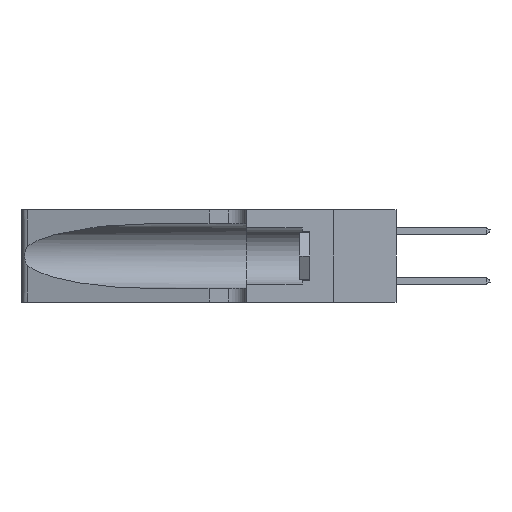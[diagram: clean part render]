
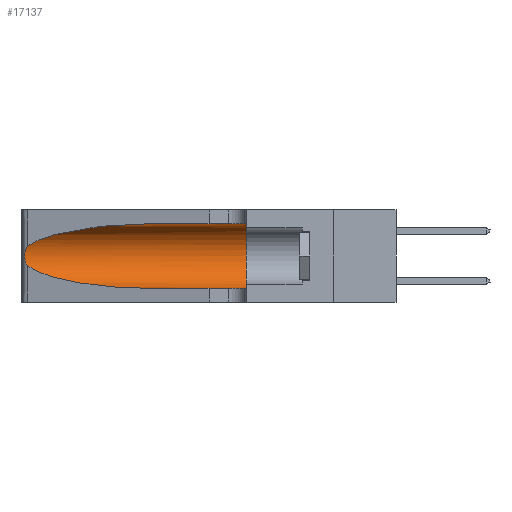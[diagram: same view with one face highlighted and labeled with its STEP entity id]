
A CAD part, left-side view. The second image highlights one B-rep face of the part: STEP entity #17137.
In plain terms, the highlighted cylindrical face has radius 3.308 mm (diameter 6.617 mm), a partial arc.
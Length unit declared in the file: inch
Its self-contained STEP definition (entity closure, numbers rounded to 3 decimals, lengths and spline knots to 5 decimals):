
#796 = ORIENTED_EDGE ( 'NONE', *, *, #6608, .F. ) ;
#1020 = CARTESIAN_POINT ( 'NONE',  ( 0.26018, 1.23835, 0.19895 ) ) ;
#1089 = CARTESIAN_POINT ( 'NONE',  ( 0.25789, 1.23486, 0.15765 ) ) ;
#1200 = ORIENTED_EDGE ( 'NONE', *, *, #15954, .F. ) ;
#2263 = EDGE_CURVE ( 'NONE', #7986, #12534, #7721, .T. ) ;
#2265 = ORIENTED_EDGE ( 'NONE', *, *, #20033, .T. ) ;
#2362 = CARTESIAN_POINT ( 'NONE',  ( 0.25487, 1.22718, 0.14631 ) ) ;
#2555 = ORIENTED_EDGE ( 'NONE', *, *, #2263, .T. ) ;
#2839 = CARTESIAN_POINT ( 'NONE',  ( 0.25487, 1.22718, 0.22369 ) ) ;
#4433 = CARTESIAN_POINT ( 'NONE',  ( 0.25639, 1.23186, 0.15144 ) ) ;
#4493 = CARTESIAN_POINT ( 'NONE',  ( 0.1305, 0.72297, 0.31525 ) ) ;
#4564 = CARTESIAN_POINT ( 'NONE',  ( 0.1305, 0.72297, 0.31525 ) ) ;
#5736 = VERTEX_POINT ( 'NONE', #21040 ) ;
#6012 = CARTESIAN_POINT ( 'NONE',  ( 0.25487, 1.22718, 0.14631 ) ) ;
#6132 = LINE ( 'NONE', #9287, #9793 ) ;
#6608 = EDGE_CURVE ( 'NONE', #20489, #16386, #6132, .T. ) ;
#6741 = CARTESIAN_POINT ( 'NONE',  ( 0.1305, 0.35, 0.185 ) ) ;
#7234 = CARTESIAN_POINT ( 'NONE',  ( 0.1305, 0.72297, 0.05475 ) ) ;
#7451 = AXIS2_PLACEMENT_3D ( 'NONE', #6741, #14644, #20525 ) ;
#7662 = ORIENTED_EDGE ( 'NONE', *, *, #10128, .T. ) ;
#7721 = LINE ( 'NONE', #16367, #12068 ) ;
#7777 = CARTESIAN_POINT ( 'NONE',  ( 0.25787, 1.23484, 0.2124 ) ) ;
#7986 = VERTEX_POINT ( 'NONE', #7234 ) ;
#9232 = CARTESIAN_POINT ( 'NONE',  ( 0.25555, 1.22994, 0.2215 ) ) ;
#9287 = CARTESIAN_POINT ( 'NONE',  ( 0.1305, 1.61858, 0.31525 ) ) ;
#9518 = CARTESIAN_POINT ( 'NONE',  ( 0.25639, 1.23184, 0.21858 ) ) ;
#9793 = VECTOR ( 'NONE', #10057, 39.37008 ) ;
#10057 = DIRECTION ( 'NONE',  ( 0., -1., 0. ) ) ;
#10128 = EDGE_CURVE ( 'NONE', #5736, #7986, #15803, .T. ) ;
#10881 = CARTESIAN_POINT ( 'NONE',  ( 0.26075, 1.23896, 0.178 ) ) ;
#11299 = CARTESIAN_POINT ( 'NONE',  ( 0.1305, 0.35, 0.31525 ) ) ;
#11866 = CARTESIAN_POINT ( 'NONE',  ( 0.1305, 1.61858, 0.185 ) ) ;
#12068 = VECTOR ( 'NONE', #21257, 39.37008 ) ;
#12501 = CARTESIAN_POINT ( 'NONE',  ( 0.25487, 1.22718, 0.22369 ) ) ;
#12534 = VERTEX_POINT ( 'NONE', #20187 ) ;
#12577 =( BOUNDED_CURVE ( )  B_SPLINE_CURVE ( 3, ( #4493, #19387, #19295, #2839 ),
 .UNSPECIFIED., .F., .F. ) 
 B_SPLINE_CURVE_WITH_KNOTS ( ( 4, 4 ),
 ( 1.5708, 2.84003 ),
 .UNSPECIFIED. ) 
 CURVE ( )  GEOMETRIC_REPRESENTATION_ITEM ( )  RATIONAL_B_SPLINE_CURVE ( ( 1., 0.87, 0.87, 1. ) ) 
 REPRESENTATION_ITEM ( '' )  );
#12721 = CARTESIAN_POINT ( 'NONE',  ( 0.25856, 1.23593, 0.16098 ) ) ;
#13360 = FACE_OUTER_BOUND ( 'NONE', #17793, .T. ) ;
#13927 = CARTESIAN_POINT ( 'NONE',  ( 0.1305, 0.72297, 0.05475 ) ) ;
#14201 = CARTESIAN_POINT ( 'NONE',  ( 0.26075, 1.23896, 0.19203 ) ) ;
#14422 = CARTESIAN_POINT ( 'NONE',  ( 0.25854, 1.2359, 0.20912 ) ) ;
#14644 = DIRECTION ( 'NONE',  ( 0., 1., 0. ) ) ;
#14737 = EDGE_CURVE ( 'NONE', #20489, #20979, #12577, .T. ) ;
#14991 = ORIENTED_EDGE ( 'NONE', *, *, #14737, .T. ) ;
#15296 = DIRECTION ( 'NONE',  ( 0., 0., -1. ) ) ;
#15533 = CARTESIAN_POINT ( 'NONE',  ( 0.25487, 1.22718, 0.22369 ) ) ;
#15803 =( BOUNDED_CURVE ( )  B_SPLINE_CURVE ( 3, ( #2362, #18840, #20323, #13927 ),
 .UNSPECIFIED., .F., .T. ) 
 B_SPLINE_CURVE_WITH_KNOTS ( ( 4, 4 ),
 ( 3.44316, 4.71239 ),
 .UNSPECIFIED. ) 
 CURVE ( )  GEOMETRIC_REPRESENTATION_ITEM ( )  RATIONAL_B_SPLINE_CURVE ( ( 1., 0.87, 0.87, 1. ) ) 
 REPRESENTATION_ITEM ( '' )  );
#15954 = EDGE_CURVE ( 'NONE', #16386, #12534, #20447, .T. ) ;
#16367 = CARTESIAN_POINT ( 'NONE',  ( 0.1305, 1.61858, 0.05475 ) ) ;
#16386 = VERTEX_POINT ( 'NONE', #11299 ) ;
#17137 = ADVANCED_FACE ( 'NONE', ( #13360 ), #19872, .F. ) ;
#17198 = B_SPLINE_CURVE_WITH_KNOTS ( 'NONE', 3,
 ( #12501, #9232, #9518, #7777, #14422, #1020, #14201, #10881, #17506, #12721, #1089, #4433, #21035, #6012 ),
 .UNSPECIFIED., .F., .F.,
 ( 4, 2, 2, 2, 2, 2, 4 ),
 ( 0., 0.00027, 0.00053, 0.00107, 0.0016, 0.00187, 0.00214 ),
 .UNSPECIFIED. ) ;
#17506 = CARTESIAN_POINT ( 'NONE',  ( 0.26017, 1.23833, 0.17102 ) ) ;
#17793 = EDGE_LOOP ( 'NONE', ( #14991, #2265, #7662, #2555, #1200, #796 ) ) ;
#18306 = DIRECTION ( 'NONE',  ( 0., -1., 0. ) ) ;
#18517 = AXIS2_PLACEMENT_3D ( 'NONE', #11866, #18306, #15296 ) ;
#18840 = CARTESIAN_POINT ( 'NONE',  ( 0.2373, 1.15595, 0.08982 ) ) ;
#19295 = CARTESIAN_POINT ( 'NONE',  ( 0.2373, 1.15595, 0.28018 ) ) ;
#19387 = CARTESIAN_POINT ( 'NONE',  ( 0.18966, 0.96281, 0.31525 ) ) ;
#19872 = CYLINDRICAL_SURFACE ( 'NONE', #18517, 0.13025 ) ;
#20033 = EDGE_CURVE ( 'NONE', #20979, #5736, #17198, .T. ) ;
#20187 = CARTESIAN_POINT ( 'NONE',  ( 0.1305, 0.35, 0.05475 ) ) ;
#20323 = CARTESIAN_POINT ( 'NONE',  ( 0.18966, 0.96281, 0.05475 ) ) ;
#20447 = CIRCLE ( 'NONE', #7451, 0.13025 ) ;
#20489 = VERTEX_POINT ( 'NONE', #4564 ) ;
#20525 = DIRECTION ( 'NONE',  ( 0., 0., 1. ) ) ;
#20979 = VERTEX_POINT ( 'NONE', #15533 ) ;
#21035 = CARTESIAN_POINT ( 'NONE',  ( 0.25555, 1.22993, 0.14849 ) ) ;
#21040 = CARTESIAN_POINT ( 'NONE',  ( 0.25487, 1.22718, 0.14631 ) ) ;
#21257 = DIRECTION ( 'NONE',  ( 0., -1., 0. ) ) ;
